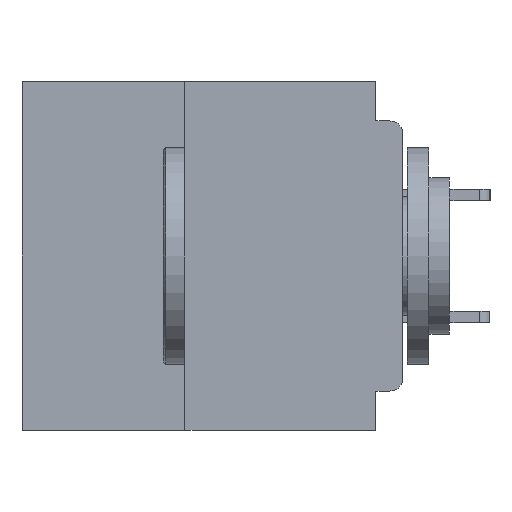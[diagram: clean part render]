
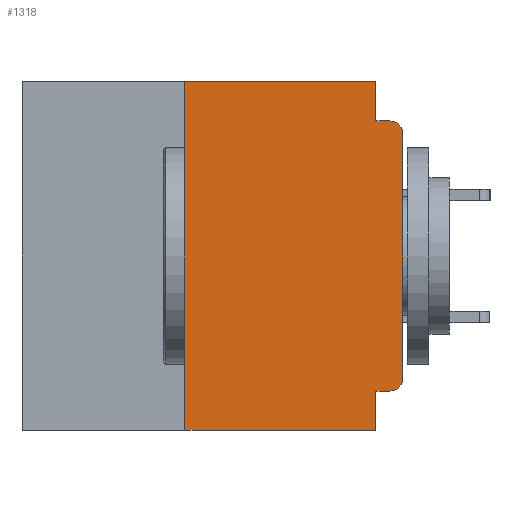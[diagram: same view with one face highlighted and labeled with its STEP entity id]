
A CAD part, left-side view. The second image highlights one B-rep face of the part: STEP entity #1318.
In plain terms, the highlighted planar face has unit normal (-1, 0, 0).
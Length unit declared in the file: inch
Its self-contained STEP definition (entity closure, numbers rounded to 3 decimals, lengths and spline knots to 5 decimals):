
#329 = CARTESIAN_POINT ( 'NONE',  ( 0., 0.25, -0.4 ) ) ;
#1318 = ADVANCED_FACE ( 'NONE', ( #15812 ), #1627, .F. ) ;
#1627 = PLANE ( 'NONE',  #20393 ) ;
#2318 = DIRECTION ( 'NONE',  ( 0., 0., -1. ) ) ;
#2323 = CARTESIAN_POINT ( 'NONE',  ( 0., 0.015, -0.045 ) ) ;
#2569 = LINE ( 'NONE', #8423, #33624 ) ;
#3174 = EDGE_CURVE ( 'NONE', #8773, #19501, #37169, .T. ) ;
#3931 = CARTESIAN_POINT ( 'NONE',  ( 0., 0., 0. ) ) ;
#4167 = LINE ( 'NONE', #28608, #26379 ) ;
#4361 = VECTOR ( 'NONE', #35817, 39.37008 ) ;
#4509 = CARTESIAN_POINT ( 'NONE',  ( 0., 0.031, -0.045 ) ) ;
#5836 = VECTOR ( 'NONE', #13613, 39.37008 ) ;
#6085 = CIRCLE ( 'NONE', #28640, 0.015 ) ;
#6510 = CARTESIAN_POINT ( 'NONE',  ( 0., 0.25, 0. ) ) ;
#6933 = ORIENTED_EDGE ( 'NONE', *, *, #7942, .T. ) ;
#7058 = DIRECTION ( 'NONE',  ( 0., 0., 1. ) ) ;
#7257 = CIRCLE ( 'NONE', #34793, 0.015 ) ;
#7942 = EDGE_CURVE ( 'NONE', #23546, #24368, #6085, .T. ) ;
#8050 = CARTESIAN_POINT ( 'NONE',  ( 0., 0.437, 0. ) ) ;
#8137 = DIRECTION ( 'NONE',  ( 0., 0., -1. ) ) ;
#8191 = DIRECTION ( 'NONE',  ( -1., 0., 0. ) ) ;
#8235 = CARTESIAN_POINT ( 'NONE',  ( 0., 0.015, -0.34 ) ) ;
#8423 = CARTESIAN_POINT ( 'NONE',  ( 0., 0.25, -0.4 ) ) ;
#8773 = VERTEX_POINT ( 'NONE', #25500 ) ;
#9810 = DIRECTION ( 'NONE',  ( 0., -1., 0. ) ) ;
#10294 = VECTOR ( 'NONE', #7058, 39.37008 ) ;
#10780 = ORIENTED_EDGE ( 'NONE', *, *, #35173, .T. ) ;
#11255 = LINE ( 'NONE', #3931, #10294 ) ;
#11940 = DIRECTION ( 'NONE',  ( 1., 0., 0. ) ) ;
#13613 = DIRECTION ( 'NONE',  ( 0., 0., -1. ) ) ;
#13816 = LINE ( 'NONE', #37348, #5836 ) ;
#14023 = ORIENTED_EDGE ( 'NONE', *, *, #27092, .F. ) ;
#14419 = DIRECTION ( 'NONE',  ( 0., 0., 1. ) ) ;
#14708 = ORIENTED_EDGE ( 'NONE', *, *, #18163, .T. ) ;
#15641 = VERTEX_POINT ( 'NONE', #4509 ) ;
#15812 = FACE_OUTER_BOUND ( 'NONE', #23805, .T. ) ;
#17331 = ORIENTED_EDGE ( 'NONE', *, *, #3174, .F. ) ;
#18163 = EDGE_CURVE ( 'NONE', #32335, #28625, #7257, .T. ) ;
#18255 = EDGE_CURVE ( 'NONE', #15641, #28625, #35308, .T. ) ;
#19041 = ORIENTED_EDGE ( 'NONE', *, *, #18255, .F. ) ;
#19501 = VERTEX_POINT ( 'NONE', #32543 ) ;
#20393 = AXIS2_PLACEMENT_3D ( 'NONE', #8050, #11940, #29595 ) ;
#20456 = DIRECTION ( 'NONE',  ( -1., 0., 0. ) ) ;
#21230 = VECTOR ( 'NONE', #9810, 39.37008 ) ;
#21341 = VECTOR ( 'NONE', #35125, 39.37008 ) ;
#21562 = VECTOR ( 'NONE', #26136, 39.37008 ) ;
#21824 = EDGE_CURVE ( 'NONE', #24485, #19501, #29598, .T. ) ;
#22293 = ORIENTED_EDGE ( 'NONE', *, *, #37154, .F. ) ;
#23546 = VERTEX_POINT ( 'NONE', #37496 ) ;
#23805 = EDGE_LOOP ( 'NONE', ( #10780, #14708, #19041, #22293, #28559, #24936, #36963, #17331, #14023, #6933 ) ) ;
#24368 = VERTEX_POINT ( 'NONE', #38221 ) ;
#24485 = VERTEX_POINT ( 'NONE', #329 ) ;
#24936 = ORIENTED_EDGE ( 'NONE', *, *, #28598, .F. ) ;
#25500 = CARTESIAN_POINT ( 'NONE',  ( 0., 0.031, -0.355 ) ) ;
#26136 = DIRECTION ( 'NONE',  ( 0., -1., 0. ) ) ;
#26379 = VECTOR ( 'NONE', #31572, 39.37008 ) ;
#27092 = EDGE_CURVE ( 'NONE', #23546, #8773, #4167, .T. ) ;
#27799 = CARTESIAN_POINT ( 'NONE',  ( 0., 0.437, 0. ) ) ;
#27912 = CARTESIAN_POINT ( 'NONE',  ( 0., 0., -0.06 ) ) ;
#28559 = ORIENTED_EDGE ( 'NONE', *, *, #38156, .F. ) ;
#28598 = EDGE_CURVE ( 'NONE', #24485, #34025, #2569, .T. ) ;
#28608 = CARTESIAN_POINT ( 'NONE',  ( 0., 0., -0.355 ) ) ;
#28625 = VERTEX_POINT ( 'NONE', #2323 ) ;
#28640 = AXIS2_PLACEMENT_3D ( 'NONE', #8235, #8191, #8137 ) ;
#29268 = LINE ( 'NONE', #27799, #21230 ) ;
#29595 = DIRECTION ( 'NONE',  ( 0., 0., -1. ) ) ;
#29598 = LINE ( 'NONE', #31980, #21562 ) ;
#31572 = DIRECTION ( 'NONE',  ( 0., 1., 0. ) ) ;
#31845 = CARTESIAN_POINT ( 'NONE',  ( 0., 0.031, 0. ) ) ;
#31906 = VERTEX_POINT ( 'NONE', #31845 ) ;
#31980 = CARTESIAN_POINT ( 'NONE',  ( 0., 0.437, -0.4 ) ) ;
#32335 = VERTEX_POINT ( 'NONE', #27912 ) ;
#32543 = CARTESIAN_POINT ( 'NONE',  ( 0., 0.031, -0.4 ) ) ;
#32890 = CARTESIAN_POINT ( 'NONE',  ( 0., 0., -0.045 ) ) ;
#33624 = VECTOR ( 'NONE', #14419, 39.37008 ) ;
#34025 = VERTEX_POINT ( 'NONE', #6510 ) ;
#34793 = AXIS2_PLACEMENT_3D ( 'NONE', #38268, #20456, #2318 ) ;
#35125 = DIRECTION ( 'NONE',  ( 0., 0., -1. ) ) ;
#35173 = EDGE_CURVE ( 'NONE', #24368, #32335, #11255, .T. ) ;
#35254 = CARTESIAN_POINT ( 'NONE',  ( 0., 0.031, -0.4 ) ) ;
#35308 = LINE ( 'NONE', #32890, #4361 ) ;
#35817 = DIRECTION ( 'NONE',  ( 0., -1., 0. ) ) ;
#36963 = ORIENTED_EDGE ( 'NONE', *, *, #21824, .T. ) ;
#37154 = EDGE_CURVE ( 'NONE', #31906, #15641, #13816, .T. ) ;
#37169 = LINE ( 'NONE', #35254, #21341 ) ;
#37348 = CARTESIAN_POINT ( 'NONE',  ( 0., 0.031, 0. ) ) ;
#37496 = CARTESIAN_POINT ( 'NONE',  ( 0., 0.015, -0.355 ) ) ;
#38156 = EDGE_CURVE ( 'NONE', #34025, #31906, #29268, .T. ) ;
#38221 = CARTESIAN_POINT ( 'NONE',  ( 0., 0., -0.34 ) ) ;
#38268 = CARTESIAN_POINT ( 'NONE',  ( 0., 0.015, -0.06 ) ) ;
